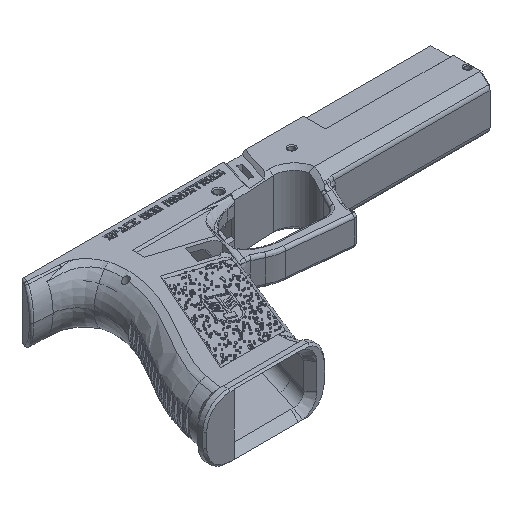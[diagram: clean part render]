
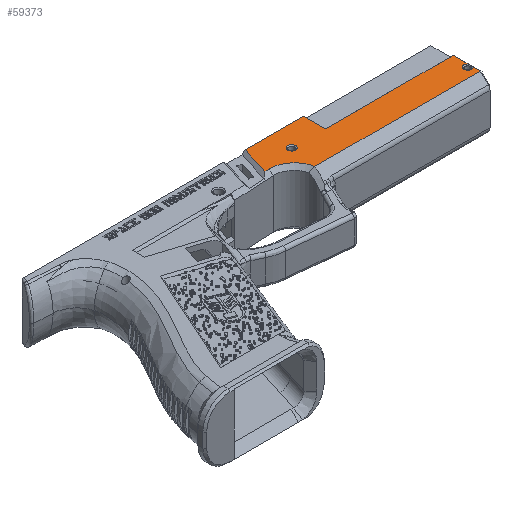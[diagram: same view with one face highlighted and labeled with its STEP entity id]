
A CAD part, isometric view. The second image highlights one B-rep face of the part: STEP entity #59373.
In plain terms, the highlighted planar face has unit normal (0, 0, 1).
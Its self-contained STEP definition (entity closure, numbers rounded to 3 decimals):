
#433=FACE_BOUND('',#16060,.T.);
#8899=PLANE('',#60706);
#12231=FACE_OUTER_BOUND('',#16059,.T.);
#16059=EDGE_LOOP('',(#54167,#54168,#54169,#54170,#54171,#54172,#54173,#54174,
#54175,#54176));
#16060=EDGE_LOOP('',(#54177));
#19602=LINE('',#134568,#23169);
#19608=LINE('',#134655,#23175);
#19634=LINE('',#135092,#23201);
#19653=LINE('',#135138,#23220);
#19655=LINE('',#135143,#23222);
#19674=LINE('',#135244,#23241);
#19675=LINE('',#135246,#23242);
#19679=LINE('',#135279,#23246);
#23169=VECTOR('',#66373,10.);
#23175=VECTOR('',#66383,10.);
#23201=VECTOR('',#66495,10.);
#23220=VECTOR('',#66522,10.);
#23222=VECTOR('',#66526,10.);
#23241=VECTOR('',#66567,10.);
#23242=VECTOR('',#66568,10.);
#23246=VECTOR('',#66600,10.);
#23416=CIRCLE('',#60052,2.025);
#23493=CIRCLE('',#60636,13.);
#23518=CIRCLE('',#60707,2.);
#26503=VERTEX_POINT('',#101574);
#29128=VERTEX_POINT('',#134564);
#29130=VERTEX_POINT('',#134567);
#29136=VERTEX_POINT('',#134650);
#29138=VERTEX_POINT('',#134660);
#29174=VERTEX_POINT('',#135089);
#29175=VERTEX_POINT('',#135091);
#29190=VERTEX_POINT('',#135136);
#29191=VERTEX_POINT('',#135140);
#29199=VERTEX_POINT('',#135234);
#29201=VERTEX_POINT('',#135245);
#33814=EDGE_CURVE('',#26503,#26503,#23416,.T.);
#37809=EDGE_CURVE('',#29128,#29130,#19602,.T.);
#37820=EDGE_CURVE('',#29136,#29128,#19608,.T.);
#37823=EDGE_CURVE('',#29138,#29136,#23493,.T.);
#37887=EDGE_CURVE('',#29174,#29175,#19634,.T.);
#37908=EDGE_CURVE('',#29190,#29175,#19653,.T.);
#37910=EDGE_CURVE('',#29191,#29138,#19655,.T.);
#37933=EDGE_CURVE('',#29199,#29191,#19674,.T.);
#37934=EDGE_CURVE('',#29190,#29201,#19675,.T.);
#37945=EDGE_CURVE('',#29201,#29199,#23518,.T.);
#37946=EDGE_CURVE('',#29130,#29174,#19679,.T.);
#54167=ORIENTED_EDGE('',*,*,#37945,.F.);
#54168=ORIENTED_EDGE('',*,*,#37934,.F.);
#54169=ORIENTED_EDGE('',*,*,#37908,.T.);
#54170=ORIENTED_EDGE('',*,*,#37887,.F.);
#54171=ORIENTED_EDGE('',*,*,#37946,.F.);
#54172=ORIENTED_EDGE('',*,*,#37809,.F.);
#54173=ORIENTED_EDGE('',*,*,#37820,.F.);
#54174=ORIENTED_EDGE('',*,*,#37823,.F.);
#54175=ORIENTED_EDGE('',*,*,#37910,.F.);
#54176=ORIENTED_EDGE('',*,*,#37933,.F.);
#54177=ORIENTED_EDGE('',*,*,#33814,.T.);
#59373=ADVANCED_FACE('',(#12231,#433),#8899,.F.);
#60052=AXIS2_PLACEMENT_3D('',#101576,#63598,#63599);
#60636=AXIS2_PLACEMENT_3D('',#134661,#66388,#66389);
#60706=AXIS2_PLACEMENT_3D('',#135277,#66596,#66597);
#60707=AXIS2_PLACEMENT_3D('',#135278,#66598,#66599);
#63598=DIRECTION('center_axis',(0.,0.,
-1.));
#63599=DIRECTION('ref_axis',(0.776,-0.63,0.));
#66373=DIRECTION('',(0.301,0.954,0.));
#66383=DIRECTION('',(-0.999,-0.055,0.));
#66388=DIRECTION('center_axis',(0.,0.,
1.));
#66389=DIRECTION('ref_axis',(0.892,-0.452,0.));
#66495=DIRECTION('',(0.,-1.,0.));
#66522=DIRECTION('',(-1.,0.,0.));
#66526=DIRECTION('',(-1.,0.,0.));
#66567=DIRECTION('',(0.,-1.,0.));
#66568=DIRECTION('',(0.,-1.,0.));
#66596=DIRECTION('center_axis',(0.,0.,
-1.));
#66597=DIRECTION('ref_axis',(0.,1.,0.));
#66598=DIRECTION('center_axis',(0.,0.,
1.));
#66599=DIRECTION('ref_axis',(-1.,0.,0.));
#66600=DIRECTION('',(1.,0.,0.));
#101574=CARTESIAN_POINT('',(97.469,-9.398,-56.855));
#101576=CARTESIAN_POINT('Origin',(95.444,-9.398,-56.855));
#134564=CARTESIAN_POINT('',(77.883,-13.165,-56.855));
#134567=CARTESIAN_POINT('',(82.591,1.767,-56.855));
#134568=CARTESIAN_POINT('',(82.185,0.48,-56.855));
#134650=CARTESIAN_POINT('',(80.217,-13.037,-56.855));
#134655=CARTESIAN_POINT('',(81.633,-12.959,-56.855));
#134660=CARTESIAN_POINT('',(93.078,-23.787,-56.855));
#134661=CARTESIAN_POINT('Origin',(80.274,-26.037,-56.855));
#135089=CARTESIAN_POINT('',(112.635,1.767,-56.855));
#135091=CARTESIAN_POINT('',(112.635,-9.733,-56.855));
#135092=CARTESIAN_POINT('',(112.635,1.513,-56.855));
#135136=CARTESIAN_POINT('',(178.635,-9.733,-56.855));
#135138=CARTESIAN_POINT('',(105.549,-9.733,-56.855));
#135140=CARTESIAN_POINT('',(178.635,-23.787,-56.855));
#135143=CARTESIAN_POINT('',(89.618,-23.787,-56.855));
#135234=CARTESIAN_POINT('',(178.635,-20.11,-56.855));
#135244=CARTESIAN_POINT('',(178.635,-25.087,-56.855));
#135245=CARTESIAN_POINT('',(178.635,-17.464,-56.855));
#135246=CARTESIAN_POINT('',(178.635,-25.087,-56.855));
#135277=CARTESIAN_POINT('Origin',(103.31,1.259,-56.855));
#135278=CARTESIAN_POINT('Origin',(177.135,-18.787,-56.855));
#135279=CARTESIAN_POINT('',(33.317,1.767,-56.855));
